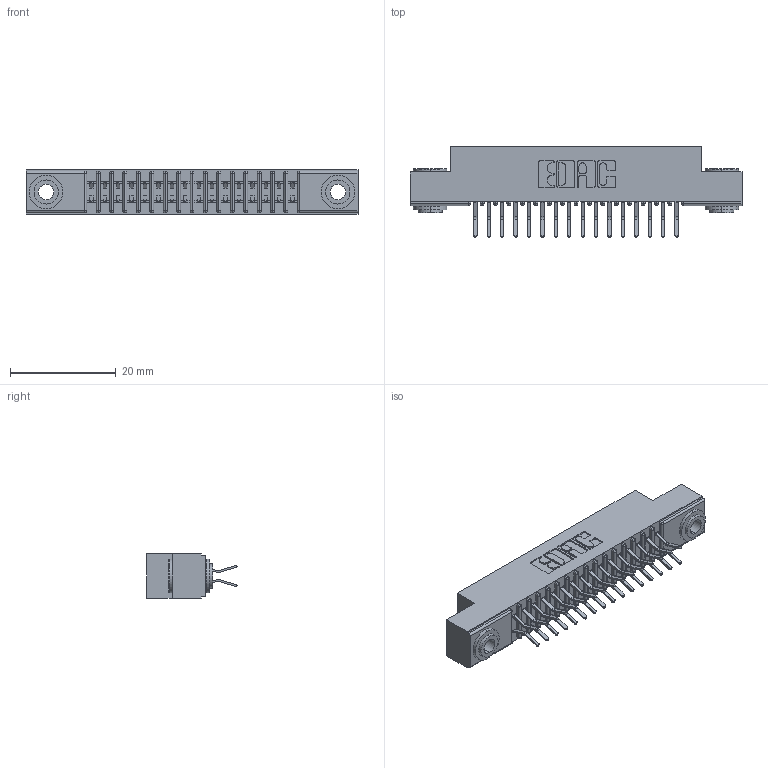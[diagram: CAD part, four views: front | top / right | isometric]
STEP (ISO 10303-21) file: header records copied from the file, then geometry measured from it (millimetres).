
FILE_DESCRIPTION (( 'STEP AP203' ), '1' );
FILE_NAME ('341-032-556-203.STEP', '2018-08-06T21:07:33', ( '' ), ( '' ), 'SwSTEP 2.0', 'SolidWorks 2016', '' );
FILE_SCHEMA (( 'CONFIG_CONTROL_DESIGN' ));
Length unit declared in the file: inch
Products named in the file (4): 341 Part_.156 (3.96) Dia Mounting Holes; 341-292-001_341-292-156; 345-250-002_345-250-002-102; 341-032-556-203
Assembly tree (35 placements, depth 2):
  341-032-556-203
    341 Part_.156 (3.96) Dia Mounting Holes
    341-292-001_341-292-156  x32
    345-250-002_345-250-002-102  x2
Bounding box: 62.87 x 17.07 x 8.38 mm (x, y, z)
Volume: 3606.8 mm3; surface area: 7460 mm2
Topology: 35 solids, 35 shells, 2408 faces, 6940 edges, 4502 vertices
Faces by surface type: plane 1372, cylinder 964, sphere 34, torus 30, cone 8
Entity records: 24032 total; most frequent: CARTESIAN_POINT 3977, ORIENTED_EDGE 3940, DIRECTION 3898, EDGE_CURVE 1970, LINE 1548, VECTOR 1548, VERTEX_POINT 1254, AXIS2_PLACEMENT_3D 1175
